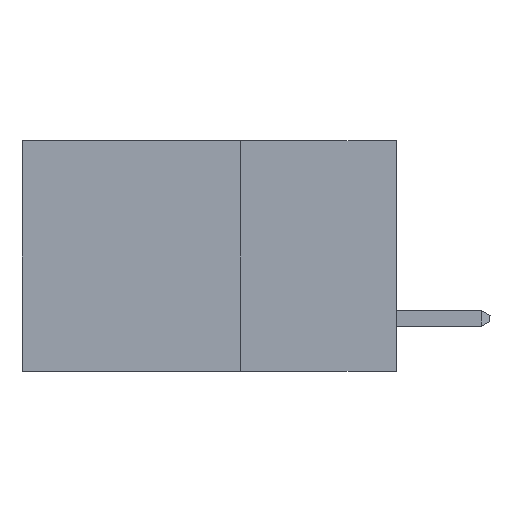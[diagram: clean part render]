
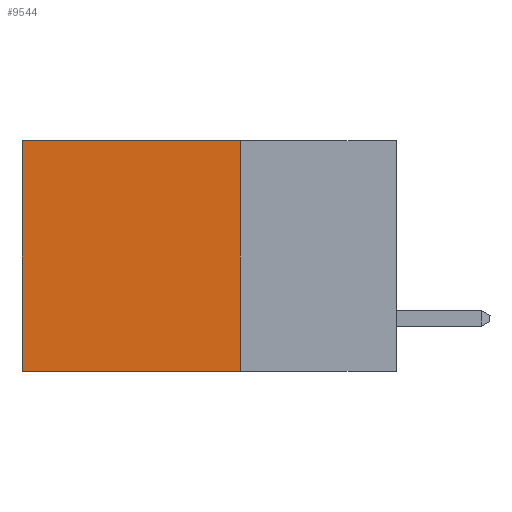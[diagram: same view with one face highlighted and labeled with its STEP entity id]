
A CAD part, left-side view. The second image highlights one B-rep face of the part: STEP entity #9544.
In plain terms, the highlighted planar face has unit normal (-1, 0, 0).
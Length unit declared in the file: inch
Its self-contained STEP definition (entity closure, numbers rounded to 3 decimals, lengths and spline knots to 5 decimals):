
#3061 = ORIENTED_EDGE ( 'NONE', *, *, #10777, .T. ) ;
#3962 = EDGE_CURVE ( 'NONE', #5237, #13241, #14906, .T. ) ;
#5237 = VERTEX_POINT ( 'NONE', #7841 ) ;
#5472 = VECTOR ( 'NONE', #17987, 39.37008 ) ;
#5842 = DIRECTION ( 'NONE',  ( 0., 0., -1. ) ) ;
#7107 = EDGE_CURVE ( 'NONE', #13015, #19515, #16773, .T. ) ;
#7420 = CARTESIAN_POINT ( 'NONE',  ( 0.2615, 0.6, -0.37 ) ) ;
#7561 = VECTOR ( 'NONE', #12401, 39.37008 ) ;
#7669 = VECTOR ( 'NONE', #11158, 39.37008 ) ;
#7841 = CARTESIAN_POINT ( 'NONE',  ( 0.2615, 0.25, 0. ) ) ;
#8169 = CARTESIAN_POINT ( 'NONE',  ( 0.2615, 0.25, -0.37 ) ) ;
#8693 = ORIENTED_EDGE ( 'NONE', *, *, #7107, .T. ) ;
#9415 = LINE ( 'NONE', #10630, #7561 ) ;
#9544 = ADVANCED_FACE ( 'NONE', ( #11251 ), #20970, .F. ) ;
#10201 = AXIS2_PLACEMENT_3D ( 'NONE', #12905, #19629, #5842 ) ;
#10361 = DIRECTION ( 'NONE',  ( 0., 0., -1. ) ) ;
#10630 = CARTESIAN_POINT ( 'NONE',  ( 0.2615, 0.25, 0. ) ) ;
#10777 = EDGE_CURVE ( 'NONE', #5237, #13015, #9415, .T. ) ;
#11158 = DIRECTION ( 'NONE',  ( 0., 1., 0. ) ) ;
#11251 = FACE_OUTER_BOUND ( 'NONE', #17815, .T. ) ;
#11920 = ORIENTED_EDGE ( 'NONE', *, *, #3962, .F. ) ;
#12401 = DIRECTION ( 'NONE',  ( 0., 1., 0. ) ) ;
#12905 = CARTESIAN_POINT ( 'NONE',  ( 0.2615, 0.25, -0.37 ) ) ;
#13015 = VERTEX_POINT ( 'NONE', #19824 ) ;
#13241 = VERTEX_POINT ( 'NONE', #16053 ) ;
#14870 = ORIENTED_EDGE ( 'NONE', *, *, #21162, .F. ) ;
#14906 = LINE ( 'NONE', #8169, #5472 ) ;
#15112 = CARTESIAN_POINT ( 'NONE',  ( 0.2615, 0.6, -0.37 ) ) ;
#16053 = CARTESIAN_POINT ( 'NONE',  ( 0.2615, 0.25, -0.37 ) ) ;
#16773 = LINE ( 'NONE', #15112, #17372 ) ;
#17372 = VECTOR ( 'NONE', #10361, 39.37008 ) ;
#17782 = LINE ( 'NONE', #21315, #7669 ) ;
#17815 = EDGE_LOOP ( 'NONE', ( #8693, #14870, #11920, #3061 ) ) ;
#17987 = DIRECTION ( 'NONE',  ( 0., 0., -1. ) ) ;
#19515 = VERTEX_POINT ( 'NONE', #7420 ) ;
#19629 = DIRECTION ( 'NONE',  ( 1., 0., 0. ) ) ;
#19824 = CARTESIAN_POINT ( 'NONE',  ( 0.2615, 0.6, 0. ) ) ;
#20970 = PLANE ( 'NONE',  #10201 ) ;
#21162 = EDGE_CURVE ( 'NONE', #13241, #19515, #17782, .T. ) ;
#21315 = CARTESIAN_POINT ( 'NONE',  ( 0.2615, 0.25, -0.37 ) ) ;
